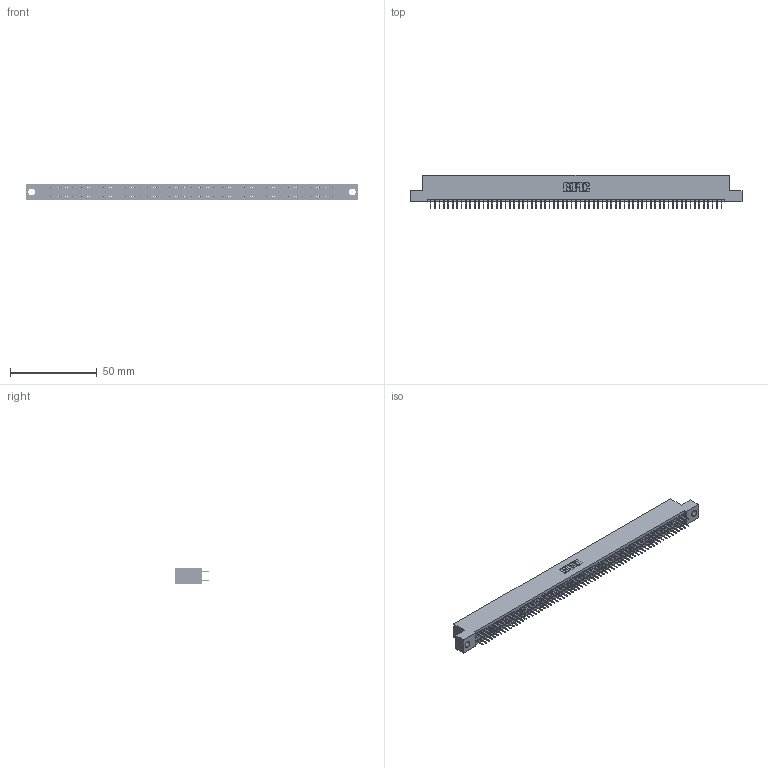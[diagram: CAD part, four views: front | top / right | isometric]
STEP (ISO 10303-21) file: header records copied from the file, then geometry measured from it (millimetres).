
FILE_DESCRIPTION (( 'STEP AP203' ), '1' );
FILE_NAME ('345-134-524-204.STEP', '2021-05-25T22:14:48', ( '' ), ( '' ), 'SwSTEP 2.0', 'SolidWorks 2020', '' );
FILE_SCHEMA (( 'CONFIG_CONTROL_DESIGN' ));
Length unit declared in the file: inch
Products named in the file (3): 345-134-524-204; 345-292-001_345-293-124; 345 Part_Flush Mounting Lugs - 0.156 Dia-TI
Assembly tree (135 placements, depth 2):
  345-134-524-204
    345 Part_Flush Mounting Lugs - 0.156 Dia-TI
    345-292-001_345-293-124  x134
Bounding box: 191.39 x 19.35 x 9.4 mm (x, y, z)
Volume: 18515 mm3; surface area: 27168.8 mm2
Topology: 135 solids, 135 shells, 7376 faces, 20879 edges, 13382 vertices
Faces by surface type: plane 5320, cylinder 2056
Entity records: 49697 total; most frequent: CARTESIAN_POINT 8310, ORIENTED_EDGE 8242, DIRECTION 7297, EDGE_CURVE 4121, LINE 3725, VECTOR 3725, VERTEX_POINT 2742, AXIS2_PLACEMENT_3D 1786
